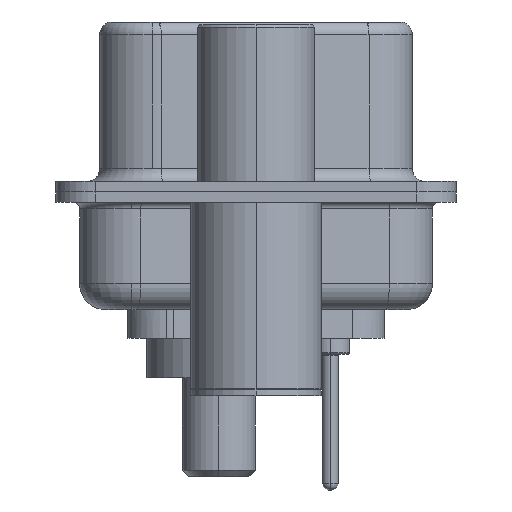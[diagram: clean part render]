
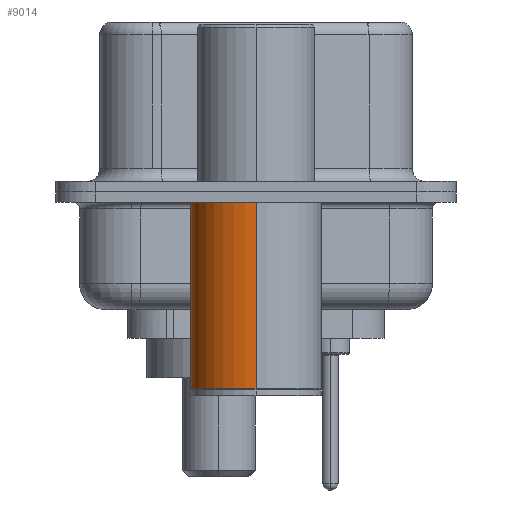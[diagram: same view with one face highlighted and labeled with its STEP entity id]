
A CAD part, left-side view. The second image highlights one B-rep face of the part: STEP entity #9014.
In plain terms, the highlighted cylindrical face has radius 2.5 mm (diameter 5 mm), a partial arc.
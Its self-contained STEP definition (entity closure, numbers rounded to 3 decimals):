
#607 = VERTEX_POINT ( 'NONE', #9710 ) ;
#962 = EDGE_CURVE ( 'NONE', #20765, #607, #8789, .T. ) ;
#1334 = CIRCLE ( 'NONE', #2124, 2.5 ) ;
#1916 = DIRECTION ( 'NONE',  ( 0., 0., 1. ) ) ;
#2124 = AXIS2_PLACEMENT_3D ( 'NONE', #20584, #7482, #7732 ) ;
#3571 = CARTESIAN_POINT ( 'NONE',  ( 2.5, 0., 0.581 ) ) ;
#3738 = CARTESIAN_POINT ( 'NONE',  ( -2.5, 0., 0.581 ) ) ;
#4048 = EDGE_LOOP ( 'NONE', ( #13633, #21704, #11354, #14239 ) ) ;
#4301 = EDGE_CURVE ( 'NONE', #16645, #21053, #1334, .T. ) ;
#4692 = VECTOR ( 'NONE', #1916, 1000. ) ;
#5234 = LINE ( 'NONE', #3738, #4692 ) ;
#5621 = CYLINDRICAL_SURFACE ( 'NONE', #10451, 2.5 ) ;
#5631 = CARTESIAN_POINT ( 'NONE',  ( 2.5, 0., -7.525 ) ) ;
#6046 = CARTESIAN_POINT ( 'NONE',  ( 0., 0., -7.525 ) ) ;
#6174 = CARTESIAN_POINT ( 'NONE',  ( -2.5, 0., -0.4 ) ) ;
#6190 = FACE_OUTER_BOUND ( 'NONE', #4048, .T. ) ;
#7091 = LINE ( 'NONE', #3571, #12437 ) ;
#7169 = DIRECTION ( 'NONE',  ( 0., 0., 1. ) ) ;
#7482 = DIRECTION ( 'NONE',  ( 0., 0., 1. ) ) ;
#7732 = DIRECTION ( 'NONE',  ( 1., 0., 0. ) ) ;
#8662 = DIRECTION ( 'NONE',  ( 1., 0., 0. ) ) ;
#8789 = CIRCLE ( 'NONE', #9915, 2.5 ) ;
#9014 = ADVANCED_FACE ( 'NONE', ( #6190 ), #5621, .T. ) ;
#9710 = CARTESIAN_POINT ( 'NONE',  ( -2.5, 0., -7.525 ) ) ;
#9915 = AXIS2_PLACEMENT_3D ( 'NONE', #6046, #18997, #8662 ) ;
#10451 = AXIS2_PLACEMENT_3D ( 'NONE', #22356, #21965, #21819 ) ;
#10561 = CARTESIAN_POINT ( 'NONE',  ( 2.5, 0., -0.4 ) ) ;
#11354 = ORIENTED_EDGE ( 'NONE', *, *, #4301, .F. ) ;
#12261 = EDGE_CURVE ( 'NONE', #607, #21053, #5234, .T. ) ;
#12437 = VECTOR ( 'NONE', #7169, 1000. ) ;
#13633 = ORIENTED_EDGE ( 'NONE', *, *, #962, .T. ) ;
#14239 = ORIENTED_EDGE ( 'NONE', *, *, #20646, .F. ) ;
#16645 = VERTEX_POINT ( 'NONE', #10561 ) ;
#18997 = DIRECTION ( 'NONE',  ( 0., 0., 1. ) ) ;
#20584 = CARTESIAN_POINT ( 'NONE',  ( 0., 0., -0.4 ) ) ;
#20646 = EDGE_CURVE ( 'NONE', #20765, #16645, #7091, .T. ) ;
#20765 = VERTEX_POINT ( 'NONE', #5631 ) ;
#21053 = VERTEX_POINT ( 'NONE', #6174 ) ;
#21704 = ORIENTED_EDGE ( 'NONE', *, *, #12261, .T. ) ;
#21819 = DIRECTION ( 'NONE',  ( 1., 0., 0. ) ) ;
#21965 = DIRECTION ( 'NONE',  ( 0., 0., 1. ) ) ;
#22356 = CARTESIAN_POINT ( 'NONE',  ( 0., 0., 0.581 ) ) ;
